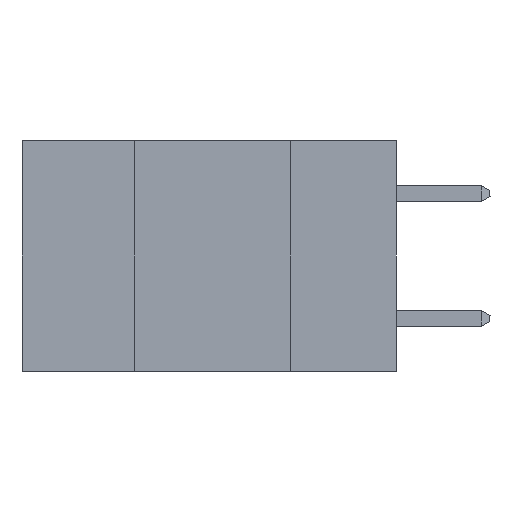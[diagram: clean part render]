
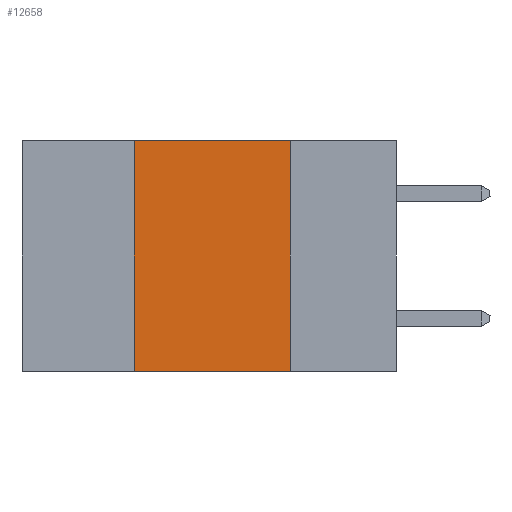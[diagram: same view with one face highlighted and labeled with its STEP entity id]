
A CAD part, left-side view. The second image highlights one B-rep face of the part: STEP entity #12658.
In plain terms, the highlighted planar face has unit normal (-1, 0, 0).
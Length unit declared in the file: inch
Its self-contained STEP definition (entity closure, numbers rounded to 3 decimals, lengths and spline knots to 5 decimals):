
#53 = CARTESIAN_POINT ( 'NONE',  ( 0., 0.42, 0. ) ) ;
#832 = LINE ( 'NONE', #7403, #11442 ) ;
#1580 = PLANE ( 'NONE',  #6495 ) ;
#1748 = EDGE_CURVE ( 'NONE', #5055, #9333, #832, .T. ) ;
#1764 = LINE ( 'NONE', #13488, #13439 ) ;
#1895 = DIRECTION ( 'NONE',  ( 0., -1., 0. ) ) ;
#2805 = CARTESIAN_POINT ( 'NONE',  ( 0., 0.6, 0. ) ) ;
#3000 = ORIENTED_EDGE ( 'NONE', *, *, #9723, .F. ) ;
#3609 = EDGE_LOOP ( 'NONE', ( #9933, #9773, #3000, #8976 ) ) ;
#4421 = VERTEX_POINT ( 'NONE', #8520 ) ;
#4958 = VECTOR ( 'NONE', #1895, 39.37008 ) ;
#5055 = VERTEX_POINT ( 'NONE', #13608 ) ;
#6495 = AXIS2_PLACEMENT_3D ( 'NONE', #2805, #11784, #12918 ) ;
#7403 = CARTESIAN_POINT ( 'NONE',  ( 0., 0.6, 0. ) ) ;
#8336 = EDGE_CURVE ( 'NONE', #4421, #11676, #10931, .T. ) ;
#8520 = CARTESIAN_POINT ( 'NONE',  ( 0., 0.42, -0.37 ) ) ;
#8544 = CARTESIAN_POINT ( 'NONE',  ( 0., 0.17, 0. ) ) ;
#8939 = VECTOR ( 'NONE', #13637, 39.37008 ) ;
#8949 = DIRECTION ( 'NONE',  ( 0., 0., -1. ) ) ;
#8976 = ORIENTED_EDGE ( 'NONE', *, *, #8336, .T. ) ;
#9333 = VERTEX_POINT ( 'NONE', #8544 ) ;
#9723 = EDGE_CURVE ( 'NONE', #4421, #5055, #14255, .T. ) ;
#9773 = ORIENTED_EDGE ( 'NONE', *, *, #1748, .F. ) ;
#9933 = ORIENTED_EDGE ( 'NONE', *, *, #14146, .F. ) ;
#10092 = FACE_OUTER_BOUND ( 'NONE', #3609, .T. ) ;
#10913 = CARTESIAN_POINT ( 'NONE',  ( 0., 0.17, -0.37 ) ) ;
#10931 = LINE ( 'NONE', #12000, #4958 ) ;
#11442 = VECTOR ( 'NONE', #14342, 39.37008 ) ;
#11676 = VERTEX_POINT ( 'NONE', #10913 ) ;
#11784 = DIRECTION ( 'NONE',  ( 1., 0., 0. ) ) ;
#12000 = CARTESIAN_POINT ( 'NONE',  ( 0., 0.6, -0.37 ) ) ;
#12658 = ADVANCED_FACE ( 'NONE', ( #10092 ), #1580, .F. ) ;
#12918 = DIRECTION ( 'NONE',  ( 0., 0., -1. ) ) ;
#13439 = VECTOR ( 'NONE', #8949, 39.37008 ) ;
#13488 = CARTESIAN_POINT ( 'NONE',  ( 0., 0.17, 0. ) ) ;
#13608 = CARTESIAN_POINT ( 'NONE',  ( 0., 0.42, 0. ) ) ;
#13637 = DIRECTION ( 'NONE',  ( 0., 0., 1. ) ) ;
#14146 = EDGE_CURVE ( 'NONE', #9333, #11676, #1764, .T. ) ;
#14255 = LINE ( 'NONE', #53, #8939 ) ;
#14342 = DIRECTION ( 'NONE',  ( 0., -1., 0. ) ) ;
